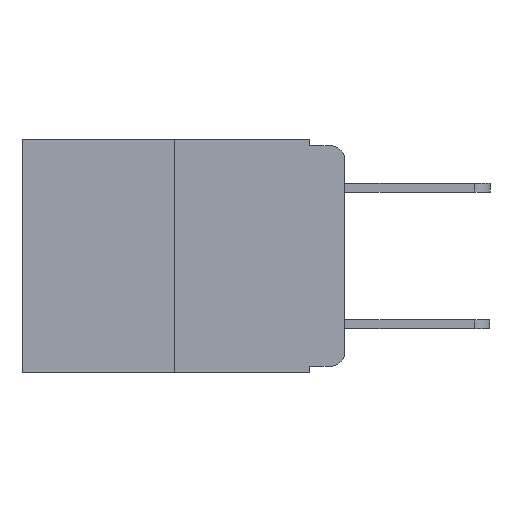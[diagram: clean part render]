
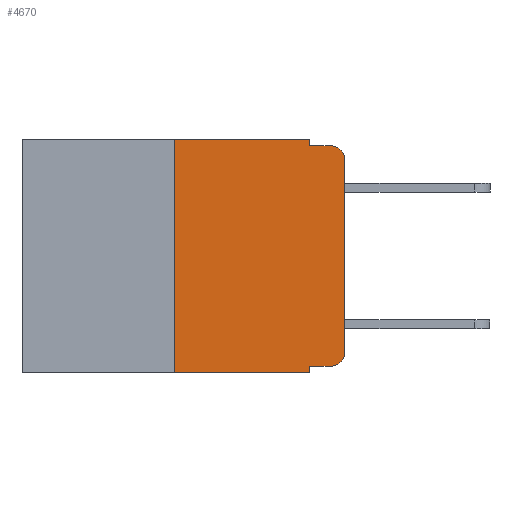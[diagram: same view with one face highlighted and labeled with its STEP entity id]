
A CAD part, left-side view. The second image highlights one B-rep face of the part: STEP entity #4670.
In plain terms, the highlighted planar face has unit normal (-1, 0, 0).
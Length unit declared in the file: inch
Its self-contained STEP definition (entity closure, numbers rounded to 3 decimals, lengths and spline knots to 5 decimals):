
#411 = EDGE_CURVE ( 'NONE', #5694, #1696, #12274, .T. ) ;
#476 = LINE ( 'NONE', #6941, #7324 ) ;
#484 = AXIS2_PLACEMENT_3D ( 'NONE', #6046, #13689, #7252 ) ;
#1288 = CARTESIAN_POINT ( 'NONE',  ( 0., 0.02, -0.01 ) ) ;
#1526 = ORIENTED_EDGE ( 'NONE', *, *, #14052, .F. ) ;
#1635 = DIRECTION ( 'NONE',  ( 0., -1., 0. ) ) ;
#1696 = VERTEX_POINT ( 'NONE', #9363 ) ;
#2273 = CARTESIAN_POINT ( 'NONE',  ( 0., 0.051, -0.01 ) ) ;
#2274 = DIRECTION ( 'NONE',  ( 0., 0., -1. ) ) ;
#2547 = VERTEX_POINT ( 'NONE', #13548 ) ;
#2651 = EDGE_LOOP ( 'NONE', ( #10576, #11579, #12552, #11075, #3877, #11096, #3708, #1526, #13760, #11996 ) ) ;
#3023 = DIRECTION ( 'NONE',  ( 0., -1., 0. ) ) ;
#3088 = CARTESIAN_POINT ( 'NONE',  ( 0., 0.051, 0. ) ) ;
#3158 = AXIS2_PLACEMENT_3D ( 'NONE', #10178, #3160, #11257 ) ;
#3160 = DIRECTION ( 'NONE',  ( -1., 0., 0. ) ) ;
#3520 = DIRECTION ( 'NONE',  ( 0., -1., 0. ) ) ;
#3639 = CARTESIAN_POINT ( 'NONE',  ( 0., 0.051, 0. ) ) ;
#3708 = ORIENTED_EDGE ( 'NONE', *, *, #6716, .T. ) ;
#3877 = ORIENTED_EDGE ( 'NONE', *, *, #7434, .F. ) ;
#4068 = EDGE_CURVE ( 'NONE', #1696, #4499, #7714, .T. ) ;
#4106 = VERTEX_POINT ( 'NONE', #11622 ) ;
#4230 = VERTEX_POINT ( 'NONE', #7399 ) ;
#4247 = DIRECTION ( 'NONE',  ( 1., 0., 0. ) ) ;
#4499 = VERTEX_POINT ( 'NONE', #1288 ) ;
#4670 = ADVANCED_FACE ( 'NONE', ( #6202 ), #11111, .F. ) ;
#4836 = CARTESIAN_POINT ( 'NONE',  ( 0., 0.051, -0.333 ) ) ;
#4941 = EDGE_CURVE ( 'NONE', #13484, #4499, #14025, .T. ) ;
#5147 = VECTOR ( 'NONE', #9426, 39.37008 ) ;
#5660 = VECTOR ( 'NONE', #10050, 39.37008 ) ;
#5694 = VERTEX_POINT ( 'NONE', #10465 ) ;
#5707 = EDGE_CURVE ( 'NONE', #2547, #13484, #13911, .T. ) ;
#5818 = CARTESIAN_POINT ( 'NONE',  ( 0., 0., -0.03 ) ) ;
#6046 = CARTESIAN_POINT ( 'NONE',  ( 0., 0.02, -0.03 ) ) ;
#6202 = FACE_OUTER_BOUND ( 'NONE', #2651, .T. ) ;
#6249 = VECTOR ( 'NONE', #7908, 39.37008 ) ;
#6378 = VERTEX_POINT ( 'NONE', #4836 ) ;
#6626 = LINE ( 'NONE', #3088, #6249 ) ;
#6633 = CARTESIAN_POINT ( 'NONE',  ( 0., 0.473, 0. ) ) ;
#6716 = EDGE_CURVE ( 'NONE', #4230, #4106, #7526, .T. ) ;
#6941 = CARTESIAN_POINT ( 'NONE',  ( 0., 0.473, 0. ) ) ;
#7252 = DIRECTION ( 'NONE',  ( 0., 0., -1. ) ) ;
#7324 = VECTOR ( 'NONE', #10336, 39.37008 ) ;
#7399 = CARTESIAN_POINT ( 'NONE',  ( 0., 0.25, -0.343 ) ) ;
#7434 = EDGE_CURVE ( 'NONE', #9130, #5694, #476, .T. ) ;
#7526 = LINE ( 'NONE', #10044, #13238 ) ;
#7714 = LINE ( 'NONE', #2273, #13410 ) ;
#7908 = DIRECTION ( 'NONE',  ( 0., 0., -1. ) ) ;
#8773 = VECTOR ( 'NONE', #2274, 39.37008 ) ;
#9130 = VERTEX_POINT ( 'NONE', #11073 ) ;
#9363 = CARTESIAN_POINT ( 'NONE',  ( 0., 0.051, -0.01 ) ) ;
#9426 = DIRECTION ( 'NONE',  ( 0., 0., 1. ) ) ;
#9523 = VECTOR ( 'NONE', #1635, 39.37008 ) ;
#9711 = CIRCLE ( 'NONE', #3158, 0.02 ) ;
#10044 = CARTESIAN_POINT ( 'NONE',  ( 0., 0.473, -0.343 ) ) ;
#10050 = DIRECTION ( 'NONE',  ( 0., 0., 1. ) ) ;
#10178 = CARTESIAN_POINT ( 'NONE',  ( 0., 0.02, -0.313 ) ) ;
#10336 = DIRECTION ( 'NONE',  ( 0., -1., 0. ) ) ;
#10465 = CARTESIAN_POINT ( 'NONE',  ( 0., 0.051, 0. ) ) ;
#10576 = ORIENTED_EDGE ( 'NONE', *, *, #5707, .T. ) ;
#11073 = CARTESIAN_POINT ( 'NONE',  ( 0., 0.25, 0. ) ) ;
#11075 = ORIENTED_EDGE ( 'NONE', *, *, #411, .F. ) ;
#11096 = ORIENTED_EDGE ( 'NONE', *, *, #14752, .F. ) ;
#11111 = PLANE ( 'NONE',  #11609 ) ;
#11257 = DIRECTION ( 'NONE',  ( 0., 0., -1. ) ) ;
#11297 = CARTESIAN_POINT ( 'NONE',  ( 0., 0.02, -0.333 ) ) ;
#11358 = VERTEX_POINT ( 'NONE', #11297 ) ;
#11579 = ORIENTED_EDGE ( 'NONE', *, *, #4941, .T. ) ;
#11609 = AXIS2_PLACEMENT_3D ( 'NONE', #6633, #4247, #12180 ) ;
#11622 = CARTESIAN_POINT ( 'NONE',  ( 0., 0.051, -0.343 ) ) ;
#11977 = LINE ( 'NONE', #12194, #5660 ) ;
#11996 = ORIENTED_EDGE ( 'NONE', *, *, #12694, .T. ) ;
#12180 = DIRECTION ( 'NONE',  ( 0., 0., -1. ) ) ;
#12194 = CARTESIAN_POINT ( 'NONE',  ( 0., 0.25, 0. ) ) ;
#12274 = LINE ( 'NONE', #3639, #8773 ) ;
#12334 = LINE ( 'NONE', #13149, #9523 ) ;
#12552 = ORIENTED_EDGE ( 'NONE', *, *, #4068, .F. ) ;
#12574 = CARTESIAN_POINT ( 'NONE',  ( 0., 0., 0. ) ) ;
#12694 = EDGE_CURVE ( 'NONE', #11358, #2547, #9711, .T. ) ;
#13149 = CARTESIAN_POINT ( 'NONE',  ( 0., 0.051, -0.333 ) ) ;
#13238 = VECTOR ( 'NONE', #3023, 39.37008 ) ;
#13357 = EDGE_CURVE ( 'NONE', #6378, #11358, #12334, .T. ) ;
#13410 = VECTOR ( 'NONE', #3520, 39.37008 ) ;
#13484 = VERTEX_POINT ( 'NONE', #5818 ) ;
#13548 = CARTESIAN_POINT ( 'NONE',  ( 0., 0., -0.313 ) ) ;
#13689 = DIRECTION ( 'NONE',  ( -1., 0., 0. ) ) ;
#13760 = ORIENTED_EDGE ( 'NONE', *, *, #13357, .T. ) ;
#13911 = LINE ( 'NONE', #12574, #5147 ) ;
#14025 = CIRCLE ( 'NONE', #484, 0.02 ) ;
#14052 = EDGE_CURVE ( 'NONE', #6378, #4106, #6626, .T. ) ;
#14752 = EDGE_CURVE ( 'NONE', #4230, #9130, #11977, .T. ) ;
